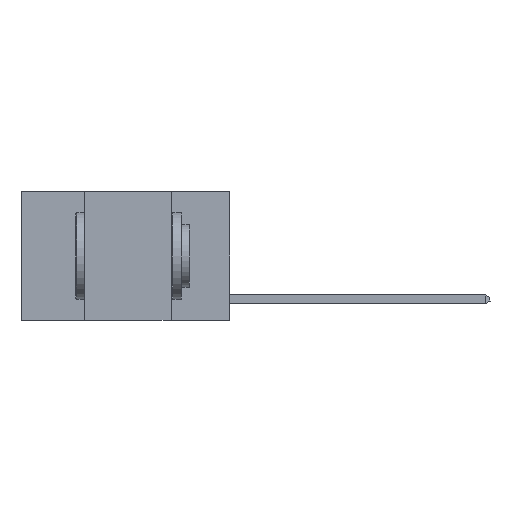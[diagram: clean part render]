
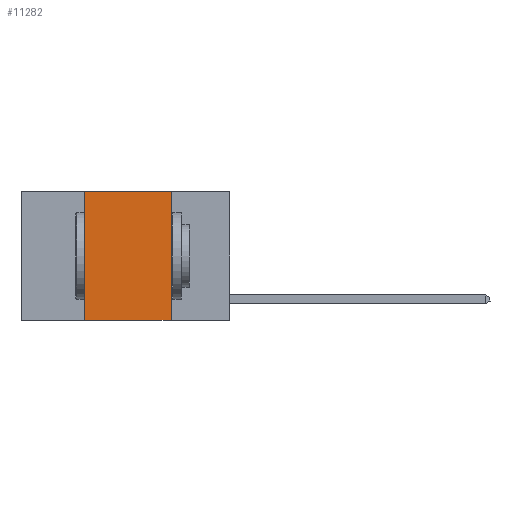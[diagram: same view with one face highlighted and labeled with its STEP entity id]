
A CAD part, left-side view. The second image highlights one B-rep face of the part: STEP entity #11282.
In plain terms, the highlighted planar face has unit normal (-1, 0, 0).
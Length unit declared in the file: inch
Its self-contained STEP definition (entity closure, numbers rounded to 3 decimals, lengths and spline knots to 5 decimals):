
#354 = EDGE_CURVE ( 'NONE', #8307, #9717, #19809, .T. ) ;
#614 = CARTESIAN_POINT ( 'NONE',  ( 0., 0.42, 0. ) ) ;
#1030 = LINE ( 'NONE', #3188, #19745 ) ;
#1070 = FACE_OUTER_BOUND ( 'NONE', #3600, .T. ) ;
#1119 = ORIENTED_EDGE ( 'NONE', *, *, #354, .F. ) ;
#1916 = CARTESIAN_POINT ( 'NONE',  ( 0., 0.17, -0.37 ) ) ;
#3054 = DIRECTION ( 'NONE',  ( 0., -1., 0. ) ) ;
#3188 = CARTESIAN_POINT ( 'NONE',  ( 0., 0.6, 0. ) ) ;
#3519 = CARTESIAN_POINT ( 'NONE',  ( 0., 0.42, 0. ) ) ;
#3567 = CARTESIAN_POINT ( 'NONE',  ( 0., 0.6, -0.37 ) ) ;
#3600 = EDGE_LOOP ( 'NONE', ( #10396, #7138, #1119, #12690 ) ) ;
#4725 = VERTEX_POINT ( 'NONE', #18879 ) ;
#5318 = DIRECTION ( 'NONE',  ( 0., -1., 0. ) ) ;
#6852 = DIRECTION ( 'NONE',  ( 1., 0., 0. ) ) ;
#6923 = DIRECTION ( 'NONE',  ( 0., 0., 1. ) ) ;
#7138 = ORIENTED_EDGE ( 'NONE', *, *, #16353, .F. ) ;
#7569 = CARTESIAN_POINT ( 'NONE',  ( 0., 0.6, 0. ) ) ;
#8307 = VERTEX_POINT ( 'NONE', #20854 ) ;
#8919 = PLANE ( 'NONE',  #10540 ) ;
#9717 = VERTEX_POINT ( 'NONE', #614 ) ;
#9894 = VERTEX_POINT ( 'NONE', #1916 ) ;
#10396 = ORIENTED_EDGE ( 'NONE', *, *, #20811, .F. ) ;
#10540 = AXIS2_PLACEMENT_3D ( 'NONE', #7569, #6852, #21519 ) ;
#10655 = DIRECTION ( 'NONE',  ( 0., 0., -1. ) ) ;
#10723 = CARTESIAN_POINT ( 'NONE',  ( 0., 0.17, 0. ) ) ;
#11282 = ADVANCED_FACE ( 'NONE', ( #1070 ), #8919, .F. ) ;
#12690 = ORIENTED_EDGE ( 'NONE', *, *, #20647, .T. ) ;
#13715 = VECTOR ( 'NONE', #5318, 39.37008 ) ;
#16353 = EDGE_CURVE ( 'NONE', #9717, #4725, #1030, .T. ) ;
#16773 = LINE ( 'NONE', #10723, #21426 ) ;
#17998 = VECTOR ( 'NONE', #6923, 39.37008 ) ;
#18567 = LINE ( 'NONE', #3567, #13715 ) ;
#18879 = CARTESIAN_POINT ( 'NONE',  ( 0., 0.17, 0. ) ) ;
#19745 = VECTOR ( 'NONE', #3054, 39.37008 ) ;
#19809 = LINE ( 'NONE', #3519, #17998 ) ;
#20647 = EDGE_CURVE ( 'NONE', #8307, #9894, #18567, .T. ) ;
#20811 = EDGE_CURVE ( 'NONE', #4725, #9894, #16773, .T. ) ;
#20854 = CARTESIAN_POINT ( 'NONE',  ( 0., 0.42, -0.37 ) ) ;
#21426 = VECTOR ( 'NONE', #10655, 39.37008 ) ;
#21519 = DIRECTION ( 'NONE',  ( 0., 0., -1. ) ) ;
